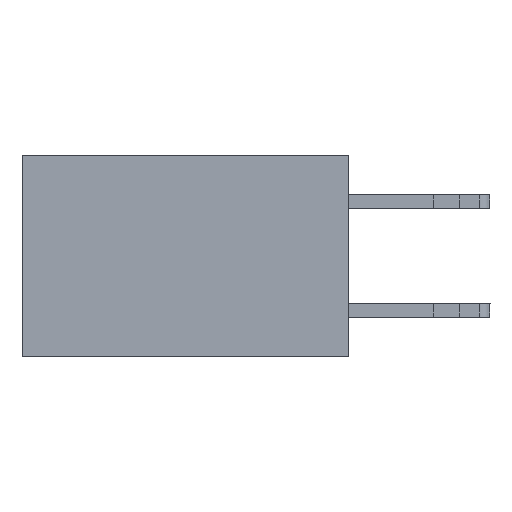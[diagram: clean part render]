
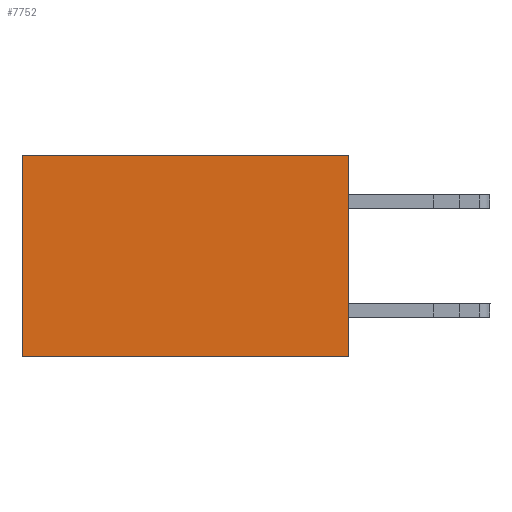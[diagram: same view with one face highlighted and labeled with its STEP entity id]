
A CAD part, left-side view. The second image highlights one B-rep face of the part: STEP entity #7752.
In plain terms, the highlighted planar face has unit normal (-1, 0, 0).
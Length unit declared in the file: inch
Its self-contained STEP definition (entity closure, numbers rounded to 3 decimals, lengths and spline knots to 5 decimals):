
#12 = VECTOR ( 'NONE', #14867, 39.37008 ) ;
#144 = ORIENTED_EDGE ( 'NONE', *, *, #11877, .T. ) ;
#170 = EDGE_LOOP ( 'NONE', ( #144, #436, #499, #723 ) ) ;
#419 = DIRECTION ( 'NONE',  ( 0., 0., -1. ) ) ;
#436 = ORIENTED_EDGE ( 'NONE', *, *, #7031, .F. ) ;
#499 = ORIENTED_EDGE ( 'NONE', *, *, #9539, .F. ) ;
#723 = ORIENTED_EDGE ( 'NONE', *, *, #13112, .T. ) ;
#1370 = CARTESIAN_POINT ( 'NONE',  ( 0.2615, 0., -0.37 ) ) ;
#2676 = DIRECTION ( 'NONE',  ( 0., 0., -1. ) ) ;
#2926 = PLANE ( 'NONE',  #13339 ) ;
#3140 = VECTOR ( 'NONE', #2676, 39.37008 ) ;
#3269 = VERTEX_POINT ( 'NONE', #8934 ) ;
#5356 = CARTESIAN_POINT ( 'NONE',  ( 0.2615, 0., -0.37 ) ) ;
#5445 = CARTESIAN_POINT ( 'NONE',  ( 0.2615, 0., -0.37 ) ) ;
#5583 = VECTOR ( 'NONE', #7876, 39.37008 ) ;
#6027 = VECTOR ( 'NONE', #6718, 39.37008 ) ;
#6526 = LINE ( 'NONE', #1370, #3140 ) ;
#6718 = DIRECTION ( 'NONE',  ( 0., 1., 0. ) ) ;
#6830 = LINE ( 'NONE', #12520, #12 ) ;
#7031 = EDGE_CURVE ( 'NONE', #14557, #13921, #15592, .T. ) ;
#7752 = ADVANCED_FACE ( 'NONE', ( #8673 ), #2926, .F. ) ;
#7876 = DIRECTION ( 'NONE',  ( 0., 1., 0. ) ) ;
#8013 = DIRECTION ( 'NONE',  ( 1., 0., 0. ) ) ;
#8673 = FACE_OUTER_BOUND ( 'NONE', #170, .T. ) ;
#8934 = CARTESIAN_POINT ( 'NONE',  ( 0.2615, 0.6, 0. ) ) ;
#9539 = EDGE_CURVE ( 'NONE', #13844, #14557, #6526, .T. ) ;
#11877 = EDGE_CURVE ( 'NONE', #3269, #13921, #6830, .T. ) ;
#12409 = LINE ( 'NONE', #13876, #5583 ) ;
#12520 = CARTESIAN_POINT ( 'NONE',  ( 0.2615, 0.6, -0.37 ) ) ;
#12798 = CARTESIAN_POINT ( 'NONE',  ( 0.2615, 0., -0.37 ) ) ;
#13112 = EDGE_CURVE ( 'NONE', #13844, #3269, #12409, .T. ) ;
#13339 = AXIS2_PLACEMENT_3D ( 'NONE', #12798, #8013, #419 ) ;
#13844 = VERTEX_POINT ( 'NONE', #15095 ) ;
#13876 = CARTESIAN_POINT ( 'NONE',  ( 0.2615, 0., 0. ) ) ;
#13921 = VERTEX_POINT ( 'NONE', #15238 ) ;
#14557 = VERTEX_POINT ( 'NONE', #5356 ) ;
#14867 = DIRECTION ( 'NONE',  ( 0., 0., -1. ) ) ;
#15095 = CARTESIAN_POINT ( 'NONE',  ( 0.2615, 0., 0. ) ) ;
#15238 = CARTESIAN_POINT ( 'NONE',  ( 0.2615, 0.6, -0.37 ) ) ;
#15592 = LINE ( 'NONE', #5445, #6027 ) ;
